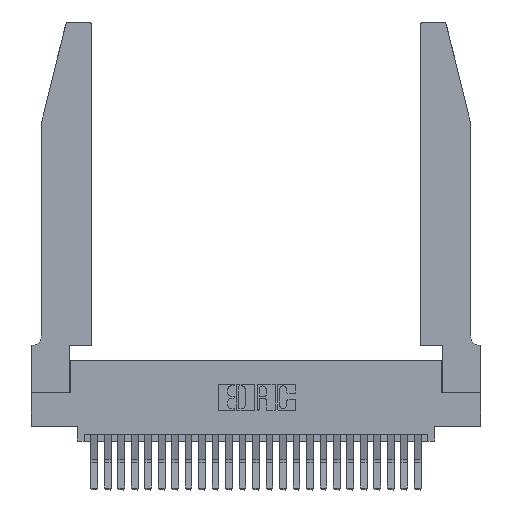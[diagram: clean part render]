
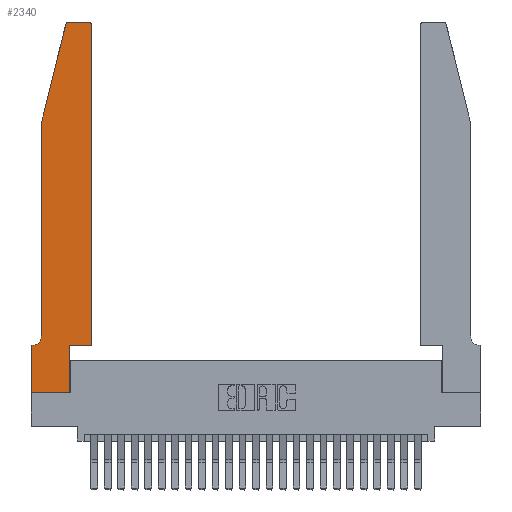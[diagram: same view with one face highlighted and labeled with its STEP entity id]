
A CAD part, top view. The second image highlights one B-rep face of the part: STEP entity #2340.
In plain terms, the highlighted planar face has unit normal (0, 0, 1).
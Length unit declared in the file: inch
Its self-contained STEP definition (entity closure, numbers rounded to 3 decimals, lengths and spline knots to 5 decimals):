
#365 = VERTEX_POINT ( 'NONE', #19305 ) ;
#452 = ORIENTED_EDGE ( 'NONE', *, *, #20013, .T. ) ;
#652 = DIRECTION ( 'NONE',  ( 0., 1., 0. ) ) ;
#840 = CARTESIAN_POINT ( 'NONE',  ( 0.25487, 2.72718, 0.37 ) ) ;
#880 = EDGE_CURVE ( 'NONE', #23801, #365, #14107, .T. ) ;
#1690 = ORIENTED_EDGE ( 'NONE', *, *, #10538, .T. ) ;
#1861 = ORIENTED_EDGE ( 'NONE', *, *, #25747, .T. ) ;
#1936 = CARTESIAN_POINT ( 'NONE',  ( 0.2605, 2.75, 0.37 ) ) ;
#2335 = LINE ( 'NONE', #4156, #21787 ) ;
#2340 = ADVANCED_FACE ( 'NONE', ( #15370 ), #2444, .T. ) ;
#2351 = AXIS2_PLACEMENT_3D ( 'NONE', #19075, #2491, #8800 ) ;
#2444 = PLANE ( 'NONE',  #26074 ) ;
#2456 = LINE ( 'NONE', #25855, #11580 ) ;
#2491 = DIRECTION ( 'NONE',  ( 0., 0., 1. ) ) ;
#2654 = EDGE_CURVE ( 'NONE', #2813, #17180, #7927, .T. ) ;
#2800 = VERTEX_POINT ( 'NONE', #840 ) ;
#2813 = VERTEX_POINT ( 'NONE', #17139 ) ;
#3239 = EDGE_CURVE ( 'NONE', #7562, #23280, #17213, .T. ) ;
#3336 = DIRECTION ( 'NONE',  ( 0., -1., 0. ) ) ;
#3344 = CARTESIAN_POINT ( 'NONE',  ( 0.2865, 0., 0.37 ) ) ;
#3379 = ORIENTED_EDGE ( 'NONE', *, *, #16169, .T. ) ;
#3650 = DIRECTION ( 'NONE',  ( 0., -1., 0. ) ) ;
#4050 = CARTESIAN_POINT ( 'NONE',  ( 0., 0., 0.37 ) ) ;
#4061 = CARTESIAN_POINT ( 'NONE',  ( 0.2865, 0.35, 0.37 ) ) ;
#4156 = CARTESIAN_POINT ( 'NONE',  ( 0.0755, 2., 0.37 ) ) ;
#4520 = VECTOR ( 'NONE', #652, 39.37008 ) ;
#4633 = DIRECTION ( 'NONE',  ( 1., 0., 0. ) ) ;
#5545 = EDGE_CURVE ( 'NONE', #365, #7562, #15223, .T. ) ;
#6079 = VERTEX_POINT ( 'NONE', #25108 ) ;
#6400 = CARTESIAN_POINT ( 'NONE',  ( 0.0755, 0.42, 0.37 ) ) ;
#6425 = DIRECTION ( 'NONE',  ( 0., 0., -1. ) ) ;
#6444 = AXIS2_PLACEMENT_3D ( 'NONE', #6794, #6425, #20884 ) ;
#6794 = CARTESIAN_POINT ( 'NONE',  ( 0.0055, 0.42, 0.37 ) ) ;
#6889 = CARTESIAN_POINT ( 'NONE',  ( 0.4205, 2.75, 0.37 ) ) ;
#7064 = EDGE_CURVE ( 'NONE', #6079, #2800, #10914, .T. ) ;
#7458 = VERTEX_POINT ( 'NONE', #6400 ) ;
#7562 = VERTEX_POINT ( 'NONE', #4050 ) ;
#7734 = CARTESIAN_POINT ( 'NONE',  ( 0., 0., 0.37 ) ) ;
#7927 = CIRCLE ( 'NONE', #17518, 0.03 ) ;
#8107 = ORIENTED_EDGE ( 'NONE', *, *, #9148, .T. ) ;
#8800 = DIRECTION ( 'NONE',  ( 1., 0., 0. ) ) ;
#8847 = CARTESIAN_POINT ( 'NONE',  ( 0., 0.35, 0.37 ) ) ;
#9148 = EDGE_CURVE ( 'NONE', #23280, #21561, #2456, .T. ) ;
#9167 = ORIENTED_EDGE ( 'NONE', *, *, #22771, .T. ) ;
#9176 = EDGE_CURVE ( 'NONE', #21561, #26867, #20602, .T. ) ;
#9745 = VECTOR ( 'NONE', #3336, 39.37008 ) ;
#10158 = VECTOR ( 'NONE', #25547, 39.37008 ) ;
#10538 = EDGE_CURVE ( 'NONE', #7458, #23801, #21829, .T. ) ;
#10594 = VECTOR ( 'NONE', #14923, 39.37008 ) ;
#10842 = CARTESIAN_POINT ( 'NONE',  ( 0.4205, 2.72, 0.37 ) ) ;
#10914 = CIRCLE ( 'NONE', #2351, 0.03 ) ;
#11516 = VECTOR ( 'NONE', #17617, 39.37008 ) ;
#11580 = VECTOR ( 'NONE', #21448, 39.37008 ) ;
#12914 = DIRECTION ( 'NONE',  ( 0., 0., 1. ) ) ;
#13028 = CARTESIAN_POINT ( 'NONE',  ( 0.0055, 0.35, 0.37 ) ) ;
#13168 = DIRECTION ( 'NONE',  ( 0., 0., 1. ) ) ;
#13307 = CARTESIAN_POINT ( 'NONE',  ( 0., 0., 0.37 ) ) ;
#13523 = VECTOR ( 'NONE', #25304, 39.37008 ) ;
#14107 = LINE ( 'NONE', #17702, #11516 ) ;
#14670 = ORIENTED_EDGE ( 'NONE', *, *, #7064, .T. ) ;
#14833 = CARTESIAN_POINT ( 'NONE',  ( 0.4505, 0.35, 0.37 ) ) ;
#14896 = LINE ( 'NONE', #25887, #4520 ) ;
#14923 = DIRECTION ( 'NONE',  ( 1., 0., 0. ) ) ;
#15223 = LINE ( 'NONE', #7734, #9745 ) ;
#15370 = FACE_OUTER_BOUND ( 'NONE', #23779, .T. ) ;
#16169 = EDGE_CURVE ( 'NONE', #17180, #6079, #19970, .T. ) ;
#16415 = VERTEX_POINT ( 'NONE', #18891 ) ;
#17139 = CARTESIAN_POINT ( 'NONE',  ( 0.4505, 2.72, 0.37 ) ) ;
#17180 = VERTEX_POINT ( 'NONE', #6889 ) ;
#17213 = LINE ( 'NONE', #13307, #10158 ) ;
#17503 = DIRECTION ( 'NONE',  ( -0.239, -0.971, 0. ) ) ;
#17518 = AXIS2_PLACEMENT_3D ( 'NONE', #10842, #12914, #21122 ) ;
#17617 = DIRECTION ( 'NONE',  ( -1., 0., 0. ) ) ;
#17702 = CARTESIAN_POINT ( 'NONE',  ( 0.0755, 0.35, 0.37 ) ) ;
#18334 = CARTESIAN_POINT ( 'NONE',  ( 0.4505, 0.35, 0.37 ) ) ;
#18891 = CARTESIAN_POINT ( 'NONE',  ( 0.0755, 2., 0.37 ) ) ;
#19075 = CARTESIAN_POINT ( 'NONE',  ( 0.284, 2.72, 0.37 ) ) ;
#19305 = CARTESIAN_POINT ( 'NONE',  ( 0., 0.35, 0.37 ) ) ;
#19970 = LINE ( 'NONE', #1936, #13523 ) ;
#20013 = EDGE_CURVE ( 'NONE', #26867, #2813, #14896, .T. ) ;
#20602 = LINE ( 'NONE', #14833, #10594 ) ;
#20884 = DIRECTION ( 'NONE',  ( -1., 0., 0. ) ) ;
#21122 = DIRECTION ( 'NONE',  ( 1., 0., 0. ) ) ;
#21448 = DIRECTION ( 'NONE',  ( 0., 1., 0. ) ) ;
#21561 = VERTEX_POINT ( 'NONE', #4061 ) ;
#21787 = VECTOR ( 'NONE', #17503, 39.37008 ) ;
#21829 = CIRCLE ( 'NONE', #6444, 0.07 ) ;
#22727 = ORIENTED_EDGE ( 'NONE', *, *, #880, .T. ) ;
#22771 = EDGE_CURVE ( 'NONE', #16415, #7458, #23887, .T. ) ;
#23048 = ORIENTED_EDGE ( 'NONE', *, *, #9176, .T. ) ;
#23280 = VERTEX_POINT ( 'NONE', #3344 ) ;
#23779 = EDGE_LOOP ( 'NONE', ( #3379, #14670, #1861, #9167, #1690, #22727, #26697, #24643, #8107, #23048, #452, #23840 ) ) ;
#23801 = VERTEX_POINT ( 'NONE', #13028 ) ;
#23840 = ORIENTED_EDGE ( 'NONE', *, *, #2654, .T. ) ;
#23887 = LINE ( 'NONE', #26241, #25538 ) ;
#24643 = ORIENTED_EDGE ( 'NONE', *, *, #3239, .T. ) ;
#25108 = CARTESIAN_POINT ( 'NONE',  ( 0.284, 2.75, 0.37 ) ) ;
#25304 = DIRECTION ( 'NONE',  ( -1., 0., 0. ) ) ;
#25538 = VECTOR ( 'NONE', #3650, 39.37008 ) ;
#25547 = DIRECTION ( 'NONE',  ( 1., 0., 0. ) ) ;
#25747 = EDGE_CURVE ( 'NONE', #2800, #16415, #2335, .T. ) ;
#25855 = CARTESIAN_POINT ( 'NONE',  ( 0.2865, 0.35, 0.37 ) ) ;
#25887 = CARTESIAN_POINT ( 'NONE',  ( 0.4505, 0.35, 0.37 ) ) ;
#26074 = AXIS2_PLACEMENT_3D ( 'NONE', #8847, #13168, #4633 ) ;
#26241 = CARTESIAN_POINT ( 'NONE',  ( 0.0755, 2., 0.37 ) ) ;
#26697 = ORIENTED_EDGE ( 'NONE', *, *, #5545, .T. ) ;
#26867 = VERTEX_POINT ( 'NONE', #18334 ) ;
